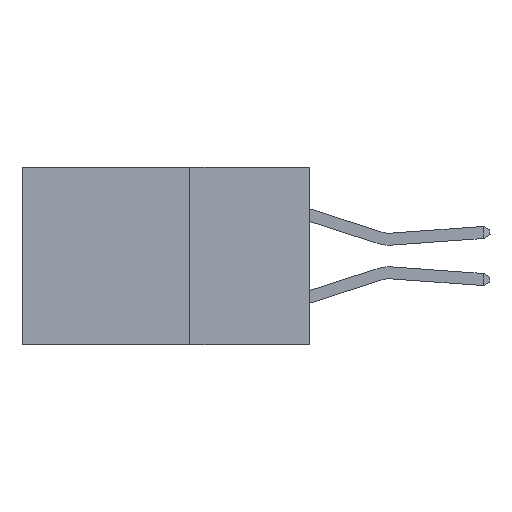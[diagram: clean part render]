
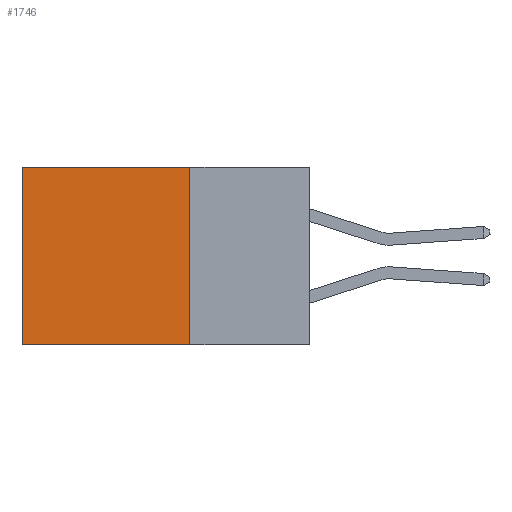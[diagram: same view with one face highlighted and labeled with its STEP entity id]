
A CAD part, left-side view. The second image highlights one B-rep face of the part: STEP entity #1746.
In plain terms, the highlighted planar face has unit normal (-1, 0, 0).
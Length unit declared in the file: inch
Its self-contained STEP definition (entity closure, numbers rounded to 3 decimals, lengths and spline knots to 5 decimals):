
#1746 = ADVANCED_FACE ( 'NONE', ( #3868 ), #11305, .F. ) ;
#2216 = DIRECTION ( 'NONE',  ( 0., 1., 0. ) ) ;
#2406 = LINE ( 'NONE', #16405, #9163 ) ;
#2535 = VERTEX_POINT ( 'NONE', #12529 ) ;
#2807 = EDGE_CURVE ( 'NONE', #5440, #3273, #12520, .T. ) ;
#3215 = AXIS2_PLACEMENT_3D ( 'NONE', #8168, #11469, #11406 ) ;
#3273 = VERTEX_POINT ( 'NONE', #16970 ) ;
#3868 = FACE_OUTER_BOUND ( 'NONE', #6507, .T. ) ;
#4048 = VECTOR ( 'NONE', #12786, 39.37008 ) ;
#4246 = EDGE_CURVE ( 'NONE', #2535, #3273, #2406, .T. ) ;
#4498 = VECTOR ( 'NONE', #14475, 39.37008 ) ;
#5440 = VERTEX_POINT ( 'NONE', #6466 ) ;
#6466 = CARTESIAN_POINT ( 'NONE',  ( 0.298, 0.6, 0. ) ) ;
#6507 = EDGE_LOOP ( 'NONE', ( #11660, #8992, #17313, #15020 ) ) ;
#8056 = CARTESIAN_POINT ( 'NONE',  ( 0.298, 0.25, 0. ) ) ;
#8168 = CARTESIAN_POINT ( 'NONE',  ( 0.298, 0.25, 0. ) ) ;
#8391 = VERTEX_POINT ( 'NONE', #8056 ) ;
#8992 = ORIENTED_EDGE ( 'NONE', *, *, #4246, .F. ) ;
#9163 = VECTOR ( 'NONE', #12378, 39.37008 ) ;
#11305 = PLANE ( 'NONE',  #3215 ) ;
#11314 = EDGE_CURVE ( 'NONE', #8391, #5440, #15994, .T. ) ;
#11406 = DIRECTION ( 'NONE',  ( 0., 0., -1. ) ) ;
#11469 = DIRECTION ( 'NONE',  ( 1., 0., 0. ) ) ;
#11574 = EDGE_CURVE ( 'NONE', #8391, #2535, #11617, .T. ) ;
#11617 = LINE ( 'NONE', #15514, #4048 ) ;
#11660 = ORIENTED_EDGE ( 'NONE', *, *, #2807, .T. ) ;
#12378 = DIRECTION ( 'NONE',  ( 0., 1., 0. ) ) ;
#12520 = LINE ( 'NONE', #14402, #4498 ) ;
#12529 = CARTESIAN_POINT ( 'NONE',  ( 0.298, 0.25, -0.37 ) ) ;
#12786 = DIRECTION ( 'NONE',  ( 0., 0., -1. ) ) ;
#14402 = CARTESIAN_POINT ( 'NONE',  ( 0.298, 0.6, 0. ) ) ;
#14475 = DIRECTION ( 'NONE',  ( 0., 0., -1. ) ) ;
#15020 = ORIENTED_EDGE ( 'NONE', *, *, #11314, .T. ) ;
#15514 = CARTESIAN_POINT ( 'NONE',  ( 0.298, 0.25, 0. ) ) ;
#15557 = VECTOR ( 'NONE', #2216, 39.37008 ) ;
#15994 = LINE ( 'NONE', #16384, #15557 ) ;
#16384 = CARTESIAN_POINT ( 'NONE',  ( 0.298, 0.25, 0. ) ) ;
#16405 = CARTESIAN_POINT ( 'NONE',  ( 0.298, 0.25, -0.37 ) ) ;
#16970 = CARTESIAN_POINT ( 'NONE',  ( 0.298, 0.6, -0.37 ) ) ;
#17313 = ORIENTED_EDGE ( 'NONE', *, *, #11574, .F. ) ;
